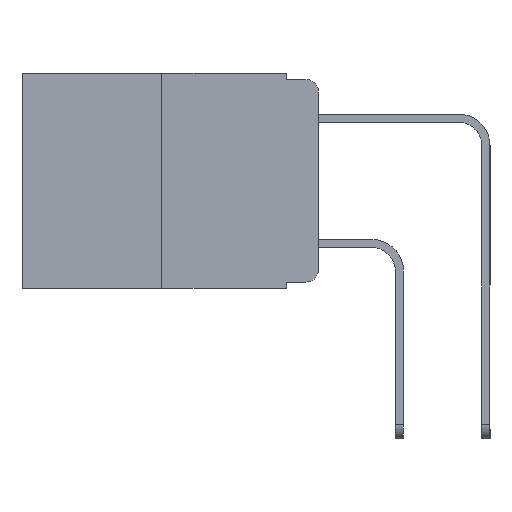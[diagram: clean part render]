
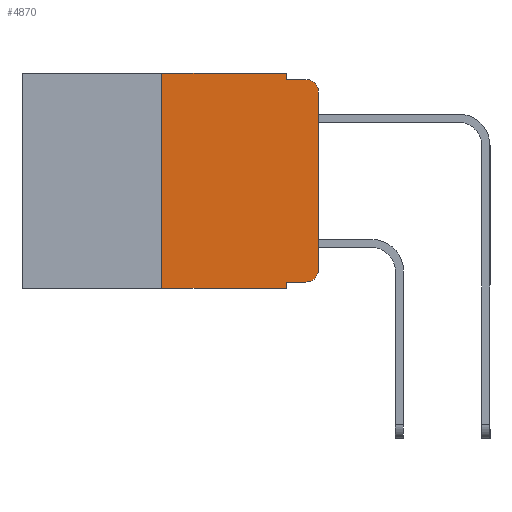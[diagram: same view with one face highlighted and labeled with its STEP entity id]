
A CAD part, left-side view. The second image highlights one B-rep face of the part: STEP entity #4870.
In plain terms, the highlighted planar face has unit normal (-1, 0, 0).
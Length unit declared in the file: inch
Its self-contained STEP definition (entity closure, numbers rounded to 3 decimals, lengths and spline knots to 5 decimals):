
#1258 = EDGE_CURVE ( 'NONE', #16023, #20911, #9296, .T. ) ;
#1480 = EDGE_CURVE ( 'NONE', #6783, #10885, #14722, .T. ) ;
#1502 = LINE ( 'NONE', #20510, #6640 ) ;
#2278 = ORIENTED_EDGE ( 'NONE', *, *, #2734, .T. ) ;
#2585 = ORIENTED_EDGE ( 'NONE', *, *, #1480, .F. ) ;
#2734 = EDGE_CURVE ( 'NONE', #22838, #16023, #17322, .T. ) ;
#2855 = CARTESIAN_POINT ( 'NONE',  ( 0., 0., -0.313 ) ) ;
#3608 = CARTESIAN_POINT ( 'NONE',  ( 0., 0., 0. ) ) ;
#3771 = LINE ( 'NONE', #12748, #15433 ) ;
#4262 = DIRECTION ( 'NONE',  ( 0., -1., 0. ) ) ;
#4373 = CARTESIAN_POINT ( 'NONE',  ( 0., 0.473, -0.343 ) ) ;
#4683 = CARTESIAN_POINT ( 'NONE',  ( 0., 0.051, -0.01 ) ) ;
#4870 = ADVANCED_FACE ( 'NONE', ( #15197 ), #7673, .F. ) ;
#5240 = CARTESIAN_POINT ( 'NONE',  ( 0., 0., -0.03 ) ) ;
#5307 = CARTESIAN_POINT ( 'NONE',  ( 0., 0.051, 0. ) ) ;
#5313 = ORIENTED_EDGE ( 'NONE', *, *, #23584, .F. ) ;
#5434 = CARTESIAN_POINT ( 'NONE',  ( 0., 0.473, 0. ) ) ;
#6031 = LINE ( 'NONE', #5307, #22615 ) ;
#6640 = VECTOR ( 'NONE', #12107, 39.37008 ) ;
#6783 = VERTEX_POINT ( 'NONE', #27253 ) ;
#6901 = ORIENTED_EDGE ( 'NONE', *, *, #19285, .F. ) ;
#7154 = DIRECTION ( 'NONE',  ( -1., 0., 0. ) ) ;
#7673 = PLANE ( 'NONE',  #27761 ) ;
#7690 = LINE ( 'NONE', #21603, #12812 ) ;
#7742 = ORIENTED_EDGE ( 'NONE', *, *, #11762, .T. ) ;
#8073 = DIRECTION ( 'NONE',  ( 0., 0., 1. ) ) ;
#9296 = CIRCLE ( 'NONE', #22302, 0.02 ) ;
#9828 = VERTEX_POINT ( 'NONE', #24048 ) ;
#9897 = DIRECTION ( 'NONE',  ( 1., 0., 0. ) ) ;
#9987 = CARTESIAN_POINT ( 'NONE',  ( 0., 0.051, -0.343 ) ) ;
#10293 = ORIENTED_EDGE ( 'NONE', *, *, #1258, .T. ) ;
#10885 = VERTEX_POINT ( 'NONE', #18857 ) ;
#11139 = DIRECTION ( 'NONE',  ( -1., 0., 0. ) ) ;
#11762 = EDGE_CURVE ( 'NONE', #9828, #22838, #19868, .T. ) ;
#12042 = ORIENTED_EDGE ( 'NONE', *, *, #25050, .F. ) ;
#12107 = DIRECTION ( 'NONE',  ( 0., 0., -1. ) ) ;
#12663 = DIRECTION ( 'NONE',  ( 0., -1., 0. ) ) ;
#12748 = CARTESIAN_POINT ( 'NONE',  ( 0., 0.051, -0.333 ) ) ;
#12812 = VECTOR ( 'NONE', #4262, 39.37008 ) ;
#14650 = EDGE_CURVE ( 'NONE', #26306, #9828, #3771, .T. ) ;
#14722 = LINE ( 'NONE', #27594, #26072 ) ;
#15197 = FACE_OUTER_BOUND ( 'NONE', #18844, .T. ) ;
#15288 = DIRECTION ( 'NONE',  ( 0., -1., 0. ) ) ;
#15418 = CARTESIAN_POINT ( 'NONE',  ( 0., 0.051, -0.333 ) ) ;
#15433 = VECTOR ( 'NONE', #12663, 39.37008 ) ;
#15445 = VECTOR ( 'NONE', #24878, 39.37008 ) ;
#16023 = VERTEX_POINT ( 'NONE', #5240 ) ;
#16599 = ORIENTED_EDGE ( 'NONE', *, *, #14650, .T. ) ;
#16790 = LINE ( 'NONE', #18428, #15445 ) ;
#16958 = DIRECTION ( 'NONE',  ( 0., -1., 0. ) ) ;
#17322 = LINE ( 'NONE', #3608, #28014 ) ;
#18428 = CARTESIAN_POINT ( 'NONE',  ( 0., 0.25, 0. ) ) ;
#18844 = EDGE_LOOP ( 'NONE', ( #2278, #10293, #12042, #5313, #2585, #27339, #22054, #6901, #16599, #7742 ) ) ;
#18857 = CARTESIAN_POINT ( 'NONE',  ( 0., 0.051, 0. ) ) ;
#19285 = EDGE_CURVE ( 'NONE', #26306, #22966, #1502, .T. ) ;
#19655 = EDGE_CURVE ( 'NONE', #23619, #22966, #21504, .T. ) ;
#19868 = CIRCLE ( 'NONE', #21758, 0.02 ) ;
#20086 = CARTESIAN_POINT ( 'NONE',  ( 0., 0.02, -0.03 ) ) ;
#20510 = CARTESIAN_POINT ( 'NONE',  ( 0., 0.051, 0. ) ) ;
#20734 = EDGE_CURVE ( 'NONE', #23619, #6783, #16790, .T. ) ;
#20911 = VERTEX_POINT ( 'NONE', #21119 ) ;
#21119 = CARTESIAN_POINT ( 'NONE',  ( 0., 0.02, -0.01 ) ) ;
#21504 = LINE ( 'NONE', #4373, #25858 ) ;
#21603 = CARTESIAN_POINT ( 'NONE',  ( 0., 0.051, -0.01 ) ) ;
#21758 = AXIS2_PLACEMENT_3D ( 'NONE', #23936, #11139, #26109 ) ;
#22054 = ORIENTED_EDGE ( 'NONE', *, *, #19655, .T. ) ;
#22265 = DIRECTION ( 'NONE',  ( 0., 0., -1. ) ) ;
#22302 = AXIS2_PLACEMENT_3D ( 'NONE', #20086, #7154, #22265 ) ;
#22615 = VECTOR ( 'NONE', #24680, 39.37008 ) ;
#22718 = CARTESIAN_POINT ( 'NONE',  ( 0., 0.25, -0.343 ) ) ;
#22838 = VERTEX_POINT ( 'NONE', #2855 ) ;
#22966 = VERTEX_POINT ( 'NONE', #9987 ) ;
#23584 = EDGE_CURVE ( 'NONE', #10885, #24552, #6031, .T. ) ;
#23619 = VERTEX_POINT ( 'NONE', #22718 ) ;
#23936 = CARTESIAN_POINT ( 'NONE',  ( 0., 0.02, -0.313 ) ) ;
#24048 = CARTESIAN_POINT ( 'NONE',  ( 0., 0.02, -0.333 ) ) ;
#24552 = VERTEX_POINT ( 'NONE', #4683 ) ;
#24680 = DIRECTION ( 'NONE',  ( 0., 0., -1. ) ) ;
#24878 = DIRECTION ( 'NONE',  ( 0., 0., 1. ) ) ;
#24910 = DIRECTION ( 'NONE',  ( 0., 0., -1. ) ) ;
#25050 = EDGE_CURVE ( 'NONE', #24552, #20911, #7690, .T. ) ;
#25858 = VECTOR ( 'NONE', #15288, 39.37008 ) ;
#26072 = VECTOR ( 'NONE', #16958, 39.37008 ) ;
#26109 = DIRECTION ( 'NONE',  ( 0., 0., -1. ) ) ;
#26306 = VERTEX_POINT ( 'NONE', #15418 ) ;
#27253 = CARTESIAN_POINT ( 'NONE',  ( 0., 0.25, 0. ) ) ;
#27339 = ORIENTED_EDGE ( 'NONE', *, *, #20734, .F. ) ;
#27594 = CARTESIAN_POINT ( 'NONE',  ( 0., 0.473, 0. ) ) ;
#27761 = AXIS2_PLACEMENT_3D ( 'NONE', #5434, #9897, #24910 ) ;
#28014 = VECTOR ( 'NONE', #8073, 39.37008 ) ;
